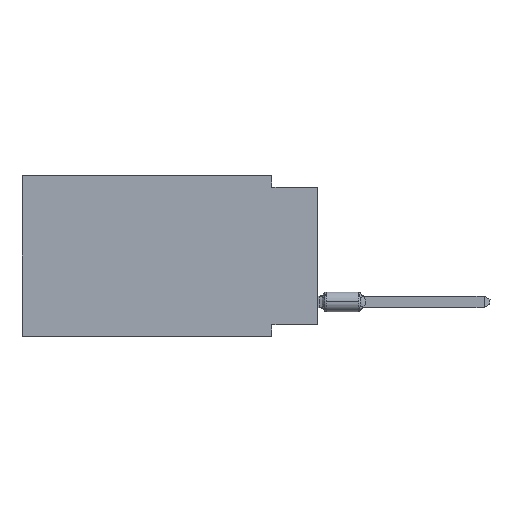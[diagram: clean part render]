
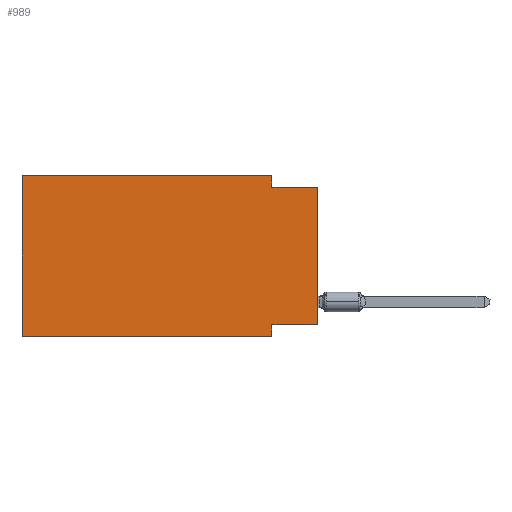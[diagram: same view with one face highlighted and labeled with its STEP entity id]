
A CAD part, left-side view. The second image highlights one B-rep face of the part: STEP entity #989.
In plain terms, the highlighted planar face has unit normal (-1, 0, 0).
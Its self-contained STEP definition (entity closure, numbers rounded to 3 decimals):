
#302 = ORIENTED_EDGE ( 'NONE', *, *, #3586, .F. ) ;
#351 = CARTESIAN_POINT ( 'NONE',  ( 0., 0., -0.635 ) ) ;
#740 = ORIENTED_EDGE ( 'NONE', *, *, #16064, .T. ) ;
#781 = CARTESIAN_POINT ( 'NONE',  ( 0., 16.383, 0. ) ) ;
#989 = ADVANCED_FACE ( 'NONE', ( #2890 ), #9784, .F. ) ;
#1072 = DIRECTION ( 'NONE',  ( 0., 0., -1. ) ) ;
#1100 = ORIENTED_EDGE ( 'NONE', *, *, #7207, .T. ) ;
#1278 = EDGE_CURVE ( 'NONE', #5915, #8074, #3599, .T. ) ;
#1317 = EDGE_CURVE ( 'NONE', #13775, #9424, #9581, .T. ) ;
#1417 = DIRECTION ( 'NONE',  ( 0., -1., 0. ) ) ;
#1529 = CARTESIAN_POINT ( 'NONE',  ( 0., 16.383, 0. ) ) ;
#1533 = DIRECTION ( 'NONE',  ( 0., -1., 0. ) ) ;
#2241 = CARTESIAN_POINT ( 'NONE',  ( 0., 2.54, 0. ) ) ;
#2433 = ORIENTED_EDGE ( 'NONE', *, *, #5009, .F. ) ;
#2613 = AXIS2_PLACEMENT_3D ( 'NONE', #1529, #8335, #15281 ) ;
#2690 = DIRECTION ( 'NONE',  ( 0., 0., 1. ) ) ;
#2890 = FACE_OUTER_BOUND ( 'NONE', #15593, .T. ) ;
#3001 = VECTOR ( 'NONE', #11131, 1000. ) ;
#3309 = CARTESIAN_POINT ( 'NONE',  ( 0., 2.54, -0.635 ) ) ;
#3586 = EDGE_CURVE ( 'NONE', #17713, #9483, #6594, .T. ) ;
#3599 = LINE ( 'NONE', #9125, #13197 ) ;
#4299 = LINE ( 'NONE', #11191, #7887 ) ;
#5009 = EDGE_CURVE ( 'NONE', #9483, #7230, #16804, .T. ) ;
#5096 = EDGE_CURVE ( 'NONE', #8074, #9222, #17769, .T. ) ;
#5413 = CARTESIAN_POINT ( 'NONE',  ( 0., 2.54, 0. ) ) ;
#5915 = VERTEX_POINT ( 'NONE', #14658 ) ;
#6294 = LINE ( 'NONE', #14781, #13374 ) ;
#6384 = ORIENTED_EDGE ( 'NONE', *, *, #9753, .F. ) ;
#6594 = LINE ( 'NONE', #2241, #13459 ) ;
#6854 = VECTOR ( 'NONE', #2690, 1000. ) ;
#7139 = ORIENTED_EDGE ( 'NONE', *, *, #5096, .F. ) ;
#7207 = EDGE_CURVE ( 'NONE', #5915, #7230, #6294, .T. ) ;
#7230 = VERTEX_POINT ( 'NONE', #11009 ) ;
#7887 = VECTOR ( 'NONE', #1417, 1000. ) ;
#8074 = VERTEX_POINT ( 'NONE', #9495 ) ;
#8335 = DIRECTION ( 'NONE',  ( 1., 0., 0. ) ) ;
#8376 = ORIENTED_EDGE ( 'NONE', *, *, #1317, .F. ) ;
#9125 = CARTESIAN_POINT ( 'NONE',  ( 0., 0., -8.255 ) ) ;
#9222 = VERTEX_POINT ( 'NONE', #14744 ) ;
#9424 = VERTEX_POINT ( 'NONE', #781 ) ;
#9483 = VERTEX_POINT ( 'NONE', #3309 ) ;
#9495 = CARTESIAN_POINT ( 'NONE',  ( 0., 2.54, -8.255 ) ) ;
#9581 = LINE ( 'NONE', #17698, #6854 ) ;
#9753 = EDGE_CURVE ( 'NONE', #9424, #17713, #4299, .T. ) ;
#9784 = PLANE ( 'NONE',  #2613 ) ;
#10652 = ORIENTED_EDGE ( 'NONE', *, *, #1278, .F. ) ;
#11009 = CARTESIAN_POINT ( 'NONE',  ( 0., 0., -0.635 ) ) ;
#11131 = DIRECTION ( 'NONE',  ( 0., -1., 0. ) ) ;
#11191 = CARTESIAN_POINT ( 'NONE',  ( 0., 16.383, 0. ) ) ;
#11987 = VECTOR ( 'NONE', #14787, 1000. ) ;
#12832 = VECTOR ( 'NONE', #1533, 1000. ) ;
#13197 = VECTOR ( 'NONE', #14626, 1000. ) ;
#13374 = VECTOR ( 'NONE', #13431, 1000. ) ;
#13431 = DIRECTION ( 'NONE',  ( 0., 0., 1. ) ) ;
#13459 = VECTOR ( 'NONE', #1072, 1000. ) ;
#13475 = LINE ( 'NONE', #17809, #3001 ) ;
#13775 = VERTEX_POINT ( 'NONE', #13830 ) ;
#13830 = CARTESIAN_POINT ( 'NONE',  ( 0., 16.383, -8.89 ) ) ;
#14626 = DIRECTION ( 'NONE',  ( 0., 1., 0. ) ) ;
#14658 = CARTESIAN_POINT ( 'NONE',  ( 0., 0., -8.255 ) ) ;
#14744 = CARTESIAN_POINT ( 'NONE',  ( 0., 2.54, -8.89 ) ) ;
#14781 = CARTESIAN_POINT ( 'NONE',  ( 0., 0., 0. ) ) ;
#14787 = DIRECTION ( 'NONE',  ( 0., 0., -1. ) ) ;
#14882 = CARTESIAN_POINT ( 'NONE',  ( 0., 2.54, -8.89 ) ) ;
#15281 = DIRECTION ( 'NONE',  ( 0., 0., -1. ) ) ;
#15593 = EDGE_LOOP ( 'NONE', ( #1100, #2433, #302, #6384, #8376, #740, #7139, #10652 ) ) ;
#16064 = EDGE_CURVE ( 'NONE', #13775, #9222, #13475, .T. ) ;
#16804 = LINE ( 'NONE', #351, #12832 ) ;
#17698 = CARTESIAN_POINT ( 'NONE',  ( 0., 16.383, 0. ) ) ;
#17713 = VERTEX_POINT ( 'NONE', #5413 ) ;
#17769 = LINE ( 'NONE', #14882, #11987 ) ;
#17809 = CARTESIAN_POINT ( 'NONE',  ( 0., 16.383, -8.89 ) ) ;
